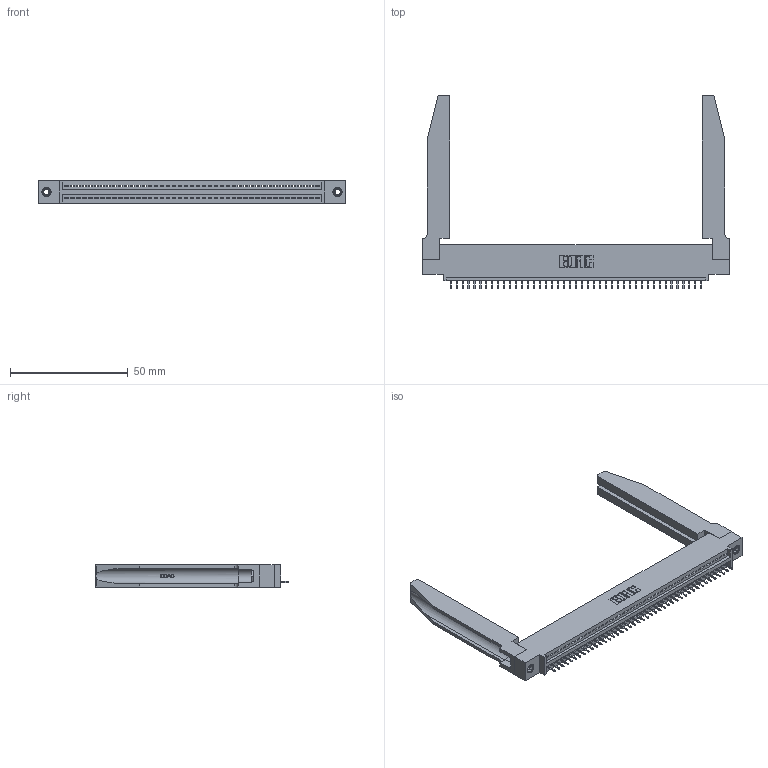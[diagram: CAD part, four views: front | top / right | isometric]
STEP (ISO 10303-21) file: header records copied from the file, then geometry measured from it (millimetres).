
FILE_DESCRIPTION (( 'STEP AP203' ), '1' );
FILE_NAME ('395-043-525-478.STEP', '2020-09-24T04:38:50', ( '' ), ( '' ), 'SwSTEP 2.0', 'SolidWorks 2020', '' );
FILE_SCHEMA (( 'CONFIG_CONTROL_DESIGN' ));
Length unit declared in the file: inch
Products named in the file (5): 395-043-525-478; 345-292-001_345-293-125; 345-250-001_345-250-001-102; 345 Part_0.110 Offset - 0.156 Dia-TH; 345-220-078_345-220-078
Assembly tree (48 placements, depth 2):
  395-043-525-478
    345 Part_0.110 Offset - 0.156 Dia-TH
    345-292-001_345-293-125  x43
    345-250-001_345-250-001-102  x2
    345-220-078_345-220-078  x2
Bounding box: 130.45 x 82.47 x 9.4 mm (x, y, z)
Volume: 19920.4 mm3; surface area: 22501.8 mm2
Topology: 48 solids, 48 shells, 3030 faces, 8701 edges, 5618 vertices
Faces by surface type: plane 2204, cylinder 774, bspline 36, cone 12, torus 4
Entity records: 37174 total; most frequent: CARTESIAN_POINT 7336, ORIENTED_EDGE 6210, DIRECTION 5413, EDGE_CURVE 3105, VECTOR 2711, LINE 2711, VERTEX_POINT 2060, AXIS2_PLACEMENT_3D 1351
